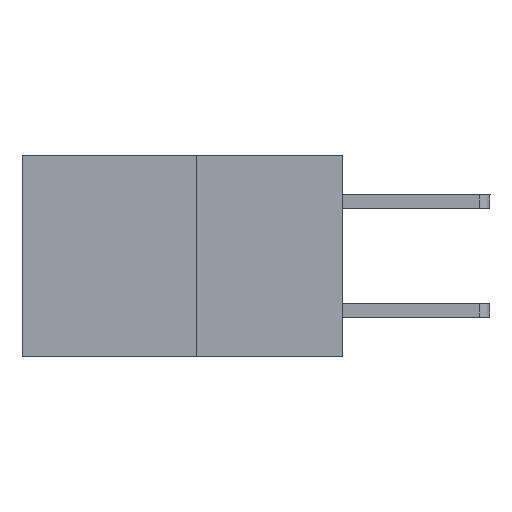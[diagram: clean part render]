
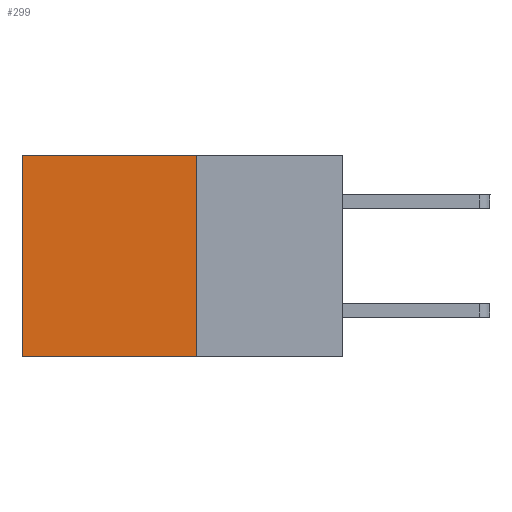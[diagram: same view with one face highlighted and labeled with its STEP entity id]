
A CAD part, left-side view. The second image highlights one B-rep face of the part: STEP entity #299.
In plain terms, the highlighted planar face has unit normal (-1, 0, 0).
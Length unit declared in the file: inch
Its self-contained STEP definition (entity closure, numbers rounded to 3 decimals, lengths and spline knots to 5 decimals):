
#18 = DIRECTION ( 'NONE',  ( 0., 1., 0. ) ) ;
#76 = CARTESIAN_POINT ( 'NONE',  ( 0.277, 0.59, -0.37 ) ) ;
#299 = ADVANCED_FACE ( 'NONE', ( #10797 ), #5553, .F. ) ;
#366 = DIRECTION ( 'NONE',  ( 0., 1., 0. ) ) ;
#468 = DIRECTION ( 'NONE',  ( 0., 0., -1. ) ) ;
#639 = DIRECTION ( 'NONE',  ( 0., 0., -1. ) ) ;
#848 = ORIENTED_EDGE ( 'NONE', *, *, #5070, .T. ) ;
#1179 = CARTESIAN_POINT ( 'NONE',  ( 0.277, 0.27, 0. ) ) ;
#2952 = VECTOR ( 'NONE', #639, 39.37008 ) ;
#3585 = ORIENTED_EDGE ( 'NONE', *, *, #8154, .T. ) ;
#3747 = CARTESIAN_POINT ( 'NONE',  ( 0.277, 0.59, 0. ) ) ;
#4014 = DIRECTION ( 'NONE',  ( 0., 0., -1. ) ) ;
#4520 = CARTESIAN_POINT ( 'NONE',  ( 0.277, 0.27, -0.37 ) ) ;
#4620 = LINE ( 'NONE', #11946, #12744 ) ;
#4955 = CARTESIAN_POINT ( 'NONE',  ( 0.277, 0.27, -0.37 ) ) ;
#5070 = EDGE_CURVE ( 'NONE', #6461, #12918, #12771, .T. ) ;
#5447 = CARTESIAN_POINT ( 'NONE',  ( 0.277, 0.27, -0.37 ) ) ;
#5553 = PLANE ( 'NONE',  #8890 ) ;
#5661 = VERTEX_POINT ( 'NONE', #76 ) ;
#6440 = VERTEX_POINT ( 'NONE', #5447 ) ;
#6461 = VERTEX_POINT ( 'NONE', #12639 ) ;
#7551 = ORIENTED_EDGE ( 'NONE', *, *, #11948, .F. ) ;
#8154 = EDGE_CURVE ( 'NONE', #12918, #5661, #8199, .T. ) ;
#8199 = LINE ( 'NONE', #11331, #12858 ) ;
#8668 = EDGE_CURVE ( 'NONE', #6461, #6440, #11242, .T. ) ;
#8712 = ORIENTED_EDGE ( 'NONE', *, *, #8668, .F. ) ;
#8890 = AXIS2_PLACEMENT_3D ( 'NONE', #4520, #9726, #468 ) ;
#9679 = VECTOR ( 'NONE', #18, 39.37008 ) ;
#9726 = DIRECTION ( 'NONE',  ( 1., 0., 0. ) ) ;
#9929 = EDGE_LOOP ( 'NONE', ( #3585, #7551, #8712, #848 ) ) ;
#10797 = FACE_OUTER_BOUND ( 'NONE', #9929, .T. ) ;
#11242 = LINE ( 'NONE', #4955, #2952 ) ;
#11331 = CARTESIAN_POINT ( 'NONE',  ( 0.277, 0.59, -0.37 ) ) ;
#11946 = CARTESIAN_POINT ( 'NONE',  ( 0.277, 0.27, -0.37 ) ) ;
#11948 = EDGE_CURVE ( 'NONE', #6440, #5661, #4620, .T. ) ;
#12639 = CARTESIAN_POINT ( 'NONE',  ( 0.277, 0.27, 0. ) ) ;
#12744 = VECTOR ( 'NONE', #366, 39.37008 ) ;
#12771 = LINE ( 'NONE', #1179, #9679 ) ;
#12858 = VECTOR ( 'NONE', #4014, 39.37008 ) ;
#12918 = VERTEX_POINT ( 'NONE', #3747 ) ;
